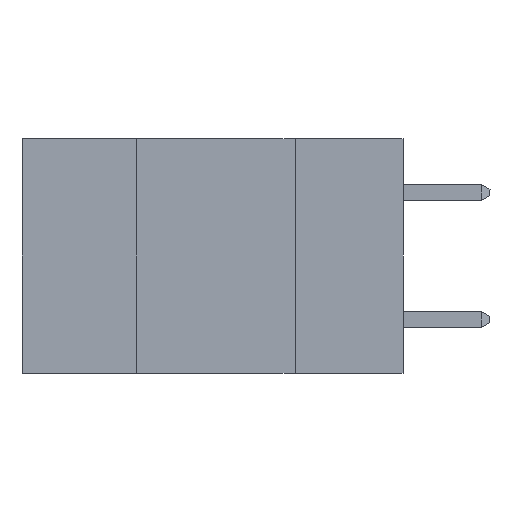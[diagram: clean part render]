
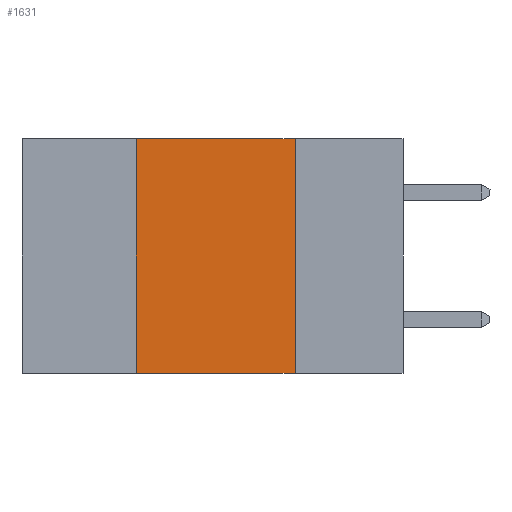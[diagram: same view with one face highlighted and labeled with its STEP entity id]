
A CAD part, left-side view. The second image highlights one B-rep face of the part: STEP entity #1631.
In plain terms, the highlighted planar face has unit normal (-1, 0, 0).
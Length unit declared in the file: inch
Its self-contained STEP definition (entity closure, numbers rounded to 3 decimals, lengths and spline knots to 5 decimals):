
#13 = VECTOR ( 'NONE', #7419, 39.37008 ) ;
#274 = VERTEX_POINT ( 'NONE', #10332 ) ;
#1529 = LINE ( 'NONE', #15028, #8437 ) ;
#1591 = CARTESIAN_POINT ( 'NONE',  ( 0., 0.17, 0. ) ) ;
#1610 = DIRECTION ( 'NONE',  ( 0., 0., 1. ) ) ;
#1631 = ADVANCED_FACE ( 'NONE', ( #5525 ), #15860, .F. ) ;
#2371 = ORIENTED_EDGE ( 'NONE', *, *, #14284, .F. ) ;
#2692 = ORIENTED_EDGE ( 'NONE', *, *, #15614, .F. ) ;
#3267 = CARTESIAN_POINT ( 'NONE',  ( 0., 0.6, -0.37 ) ) ;
#3835 = DIRECTION ( 'NONE',  ( 0., 0., -1. ) ) ;
#4185 = LINE ( 'NONE', #3267, #13 ) ;
#4234 = DIRECTION ( 'NONE',  ( 0., -1., 0. ) ) ;
#4516 = EDGE_CURVE ( 'NONE', #5470, #274, #4185, .T. ) ;
#5470 = VERTEX_POINT ( 'NONE', #16343 ) ;
#5509 = CARTESIAN_POINT ( 'NONE',  ( 0., 0.6, 0. ) ) ;
#5525 = FACE_OUTER_BOUND ( 'NONE', #8639, .T. ) ;
#6836 = CARTESIAN_POINT ( 'NONE',  ( 0., 0.17, 0. ) ) ;
#7144 = LINE ( 'NONE', #6836, #13880 ) ;
#7419 = DIRECTION ( 'NONE',  ( 0., -1., 0. ) ) ;
#7427 = VERTEX_POINT ( 'NONE', #1591 ) ;
#7844 = AXIS2_PLACEMENT_3D ( 'NONE', #13226, #11949, #3835 ) ;
#8239 = DIRECTION ( 'NONE',  ( 0., 0., -1. ) ) ;
#8437 = VECTOR ( 'NONE', #1610, 39.37008 ) ;
#8639 = EDGE_LOOP ( 'NONE', ( #2692, #2371, #10958, #13020 ) ) ;
#8742 = EDGE_CURVE ( 'NONE', #5470, #16624, #1529, .T. ) ;
#10332 = CARTESIAN_POINT ( 'NONE',  ( 0., 0.17, -0.37 ) ) ;
#10958 = ORIENTED_EDGE ( 'NONE', *, *, #8742, .F. ) ;
#11258 = VECTOR ( 'NONE', #4234, 39.37008 ) ;
#11949 = DIRECTION ( 'NONE',  ( 1., 0., 0. ) ) ;
#13020 = ORIENTED_EDGE ( 'NONE', *, *, #4516, .T. ) ;
#13226 = CARTESIAN_POINT ( 'NONE',  ( 0., 0.6, 0. ) ) ;
#13880 = VECTOR ( 'NONE', #8239, 39.37008 ) ;
#14284 = EDGE_CURVE ( 'NONE', #16624, #7427, #15151, .T. ) ;
#14320 = CARTESIAN_POINT ( 'NONE',  ( 0., 0.42, 0. ) ) ;
#15028 = CARTESIAN_POINT ( 'NONE',  ( 0., 0.42, 0. ) ) ;
#15151 = LINE ( 'NONE', #5509, #11258 ) ;
#15614 = EDGE_CURVE ( 'NONE', #7427, #274, #7144, .T. ) ;
#15860 = PLANE ( 'NONE',  #7844 ) ;
#16343 = CARTESIAN_POINT ( 'NONE',  ( 0., 0.42, -0.37 ) ) ;
#16624 = VERTEX_POINT ( 'NONE', #14320 ) ;
